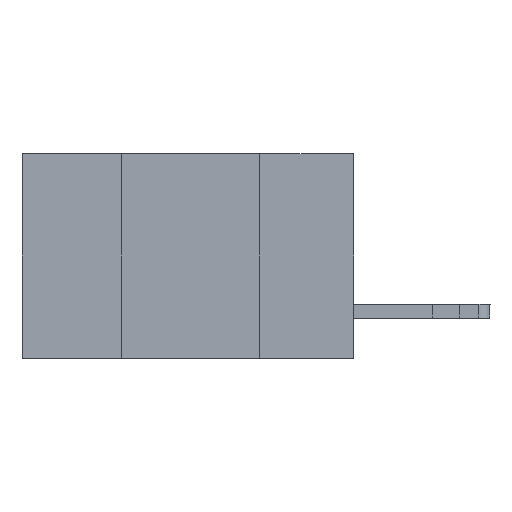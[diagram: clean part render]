
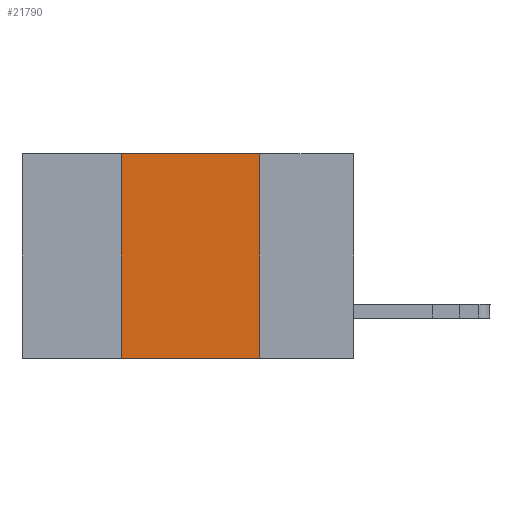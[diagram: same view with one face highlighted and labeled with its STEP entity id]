
A CAD part, left-side view. The second image highlights one B-rep face of the part: STEP entity #21790.
In plain terms, the highlighted planar face has unit normal (-1, 0, 0).
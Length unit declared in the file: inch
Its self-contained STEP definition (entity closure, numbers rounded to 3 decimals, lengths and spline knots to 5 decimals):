
#308 = LINE ( 'NONE', #1077, #17914 ) ;
#374 = DIRECTION ( 'NONE',  ( 0., 0., -1. ) ) ;
#413 = VECTOR ( 'NONE', #9909, 39.37008 ) ;
#1077 = CARTESIAN_POINT ( 'NONE',  ( 0., 0.6, -0.37 ) ) ;
#1743 = ORIENTED_EDGE ( 'NONE', *, *, #15140, .F. ) ;
#2779 = VECTOR ( 'NONE', #21264, 39.37008 ) ;
#2808 = ORIENTED_EDGE ( 'NONE', *, *, #16883, .F. ) ;
#4978 = CARTESIAN_POINT ( 'NONE',  ( 0., 0.17, 0. ) ) ;
#5561 = CARTESIAN_POINT ( 'NONE',  ( 0., 0.17, -0.37 ) ) ;
#5994 = LINE ( 'NONE', #16560, #413 ) ;
#6339 = PLANE ( 'NONE',  #9660 ) ;
#6728 = CARTESIAN_POINT ( 'NONE',  ( 0., 0.42, -0.37 ) ) ;
#7460 = VERTEX_POINT ( 'NONE', #13348 ) ;
#8232 = DIRECTION ( 'NONE',  ( 1., 0., 0. ) ) ;
#8311 = LINE ( 'NONE', #17515, #2779 ) ;
#9660 = AXIS2_PLACEMENT_3D ( 'NONE', #21512, #8232, #18042 ) ;
#9909 = DIRECTION ( 'NONE',  ( 0., -1., 0. ) ) ;
#9955 = VECTOR ( 'NONE', #374, 39.37008 ) ;
#12670 = VERTEX_POINT ( 'NONE', #6728 ) ;
#13348 = CARTESIAN_POINT ( 'NONE',  ( 0., 0.42, 0. ) ) ;
#13801 = EDGE_CURVE ( 'NONE', #21292, #16337, #13865, .T. ) ;
#13865 = LINE ( 'NONE', #20316, #9955 ) ;
#15140 = EDGE_CURVE ( 'NONE', #12670, #7460, #8311, .T. ) ;
#15756 = FACE_OUTER_BOUND ( 'NONE', #17429, .T. ) ;
#15850 = ORIENTED_EDGE ( 'NONE', *, *, #19913, .T. ) ;
#16337 = VERTEX_POINT ( 'NONE', #5561 ) ;
#16560 = CARTESIAN_POINT ( 'NONE',  ( 0., 0.6, 0. ) ) ;
#16883 = EDGE_CURVE ( 'NONE', #7460, #21292, #5994, .T. ) ;
#17429 = EDGE_LOOP ( 'NONE', ( #19240, #2808, #1743, #15850 ) ) ;
#17515 = CARTESIAN_POINT ( 'NONE',  ( 0., 0.42, 0. ) ) ;
#17746 = DIRECTION ( 'NONE',  ( 0., -1., 0. ) ) ;
#17914 = VECTOR ( 'NONE', #17746, 39.37008 ) ;
#18042 = DIRECTION ( 'NONE',  ( 0., 0., -1. ) ) ;
#19240 = ORIENTED_EDGE ( 'NONE', *, *, #13801, .F. ) ;
#19913 = EDGE_CURVE ( 'NONE', #12670, #16337, #308, .T. ) ;
#20316 = CARTESIAN_POINT ( 'NONE',  ( 0., 0.17, 0. ) ) ;
#21264 = DIRECTION ( 'NONE',  ( 0., 0., 1. ) ) ;
#21292 = VERTEX_POINT ( 'NONE', #4978 ) ;
#21512 = CARTESIAN_POINT ( 'NONE',  ( 0., 0.6, 0. ) ) ;
#21790 = ADVANCED_FACE ( 'NONE', ( #15756 ), #6339, .F. ) ;
